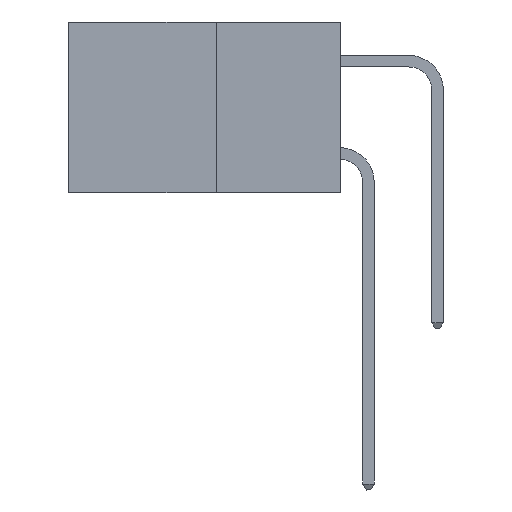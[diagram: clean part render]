
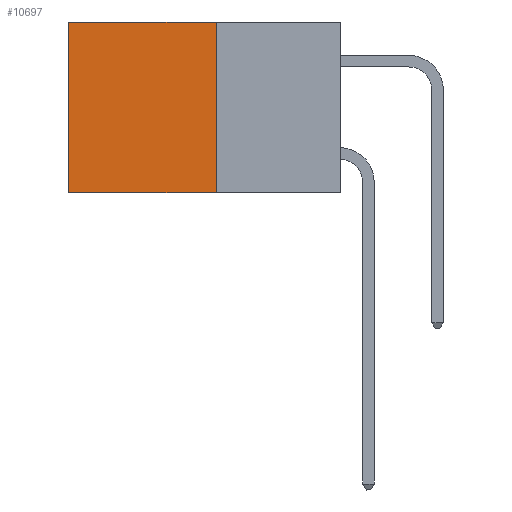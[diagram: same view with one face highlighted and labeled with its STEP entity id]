
A CAD part, left-side view. The second image highlights one B-rep face of the part: STEP entity #10697.
In plain terms, the highlighted planar face has unit normal (-1, 0, 0).
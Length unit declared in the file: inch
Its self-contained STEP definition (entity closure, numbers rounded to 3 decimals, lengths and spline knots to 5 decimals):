
#71 = CARTESIAN_POINT ( 'NONE',  ( 0.277, 0.27, -0.37 ) ) ;
#1473 = LINE ( 'NONE', #1853, #23205 ) ;
#1853 = CARTESIAN_POINT ( 'NONE',  ( 0.277, 0.27, 0. ) ) ;
#3124 = DIRECTION ( 'NONE',  ( 0., 0., -1. ) ) ;
#3174 = CARTESIAN_POINT ( 'NONE',  ( 0.277, 0.27, -0.37 ) ) ;
#4634 = EDGE_CURVE ( 'NONE', #28449, #13125, #16898, .T. ) ;
#5163 = ORIENTED_EDGE ( 'NONE', *, *, #4634, .F. ) ;
#5419 = VERTEX_POINT ( 'NONE', #6026 ) ;
#5837 = DIRECTION ( 'NONE',  ( 1., 0., 0. ) ) ;
#6026 = CARTESIAN_POINT ( 'NONE',  ( 0.277, 0.59, -0.37 ) ) ;
#7726 = EDGE_LOOP ( 'NONE', ( #34530, #19746, #5163, #36073 ) ) ;
#8363 = AXIS2_PLACEMENT_3D ( 'NONE', #71, #5837, #25600 ) ;
#9383 = VECTOR ( 'NONE', #3124, 39.37008 ) ;
#10361 = DIRECTION ( 'NONE',  ( 0., 1., 0. ) ) ;
#10451 = VECTOR ( 'NONE', #25396, 39.37008 ) ;
#10697 = ADVANCED_FACE ( 'NONE', ( #19880 ), #22774, .F. ) ;
#11333 = LINE ( 'NONE', #11351, #10451 ) ;
#11351 = CARTESIAN_POINT ( 'NONE',  ( 0.277, 0.27, -0.37 ) ) ;
#12062 = VERTEX_POINT ( 'NONE', #17027 ) ;
#12594 = CARTESIAN_POINT ( 'NONE',  ( 0.277, 0.59, -0.37 ) ) ;
#13125 = VERTEX_POINT ( 'NONE', #13394 ) ;
#13394 = CARTESIAN_POINT ( 'NONE',  ( 0.277, 0.27, -0.37 ) ) ;
#15440 = DIRECTION ( 'NONE',  ( 0., 0., -1. ) ) ;
#16898 = LINE ( 'NONE', #3174, #9383 ) ;
#17027 = CARTESIAN_POINT ( 'NONE',  ( 0.277, 0.59, 0. ) ) ;
#17848 = EDGE_CURVE ( 'NONE', #13125, #5419, #11333, .T. ) ;
#19035 = VECTOR ( 'NONE', #15440, 39.37008 ) ;
#19746 = ORIENTED_EDGE ( 'NONE', *, *, #17848, .F. ) ;
#19880 = FACE_OUTER_BOUND ( 'NONE', #7726, .T. ) ;
#19908 = LINE ( 'NONE', #12594, #19035 ) ;
#22009 = EDGE_CURVE ( 'NONE', #12062, #5419, #19908, .T. ) ;
#22774 = PLANE ( 'NONE',  #8363 ) ;
#23205 = VECTOR ( 'NONE', #10361, 39.37008 ) ;
#25396 = DIRECTION ( 'NONE',  ( 0., 1., 0. ) ) ;
#25600 = DIRECTION ( 'NONE',  ( 0., 0., -1. ) ) ;
#28449 = VERTEX_POINT ( 'NONE', #35071 ) ;
#34530 = ORIENTED_EDGE ( 'NONE', *, *, #22009, .T. ) ;
#35071 = CARTESIAN_POINT ( 'NONE',  ( 0.277, 0.27, 0. ) ) ;
#35742 = EDGE_CURVE ( 'NONE', #28449, #12062, #1473, .T. ) ;
#36073 = ORIENTED_EDGE ( 'NONE', *, *, #35742, .T. ) ;
